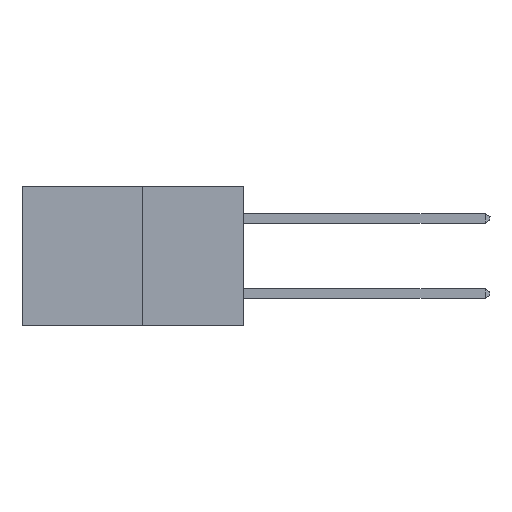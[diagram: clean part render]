
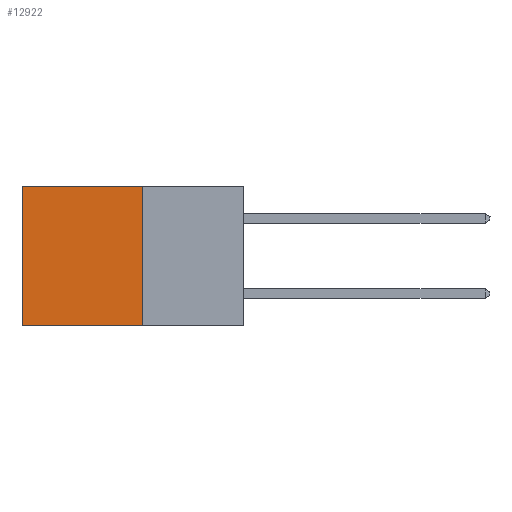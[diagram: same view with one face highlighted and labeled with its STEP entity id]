
A CAD part, left-side view. The second image highlights one B-rep face of the part: STEP entity #12922.
In plain terms, the highlighted planar face has unit normal (-1, 0, 0).
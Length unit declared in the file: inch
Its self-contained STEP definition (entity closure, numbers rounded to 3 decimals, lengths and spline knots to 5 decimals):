
#320 = AXIS2_PLACEMENT_3D ( 'NONE', #5425, #6801, #15968 ) ;
#553 = VERTEX_POINT ( 'NONE', #7725 ) ;
#2190 = CARTESIAN_POINT ( 'NONE',  ( 0.277, 0.27, -0.37 ) ) ;
#2912 = EDGE_CURVE ( 'NONE', #14401, #6390, #11120, .T. ) ;
#3602 = EDGE_CURVE ( 'NONE', #6390, #7229, #11902, .T. ) ;
#4695 = CARTESIAN_POINT ( 'NONE',  ( 0.277, 0.59, -0.37 ) ) ;
#5425 = CARTESIAN_POINT ( 'NONE',  ( 0.277, 0.27, -0.37 ) ) ;
#6149 = CARTESIAN_POINT ( 'NONE',  ( 0.277, 0.59, 0. ) ) ;
#6390 = VERTEX_POINT ( 'NONE', #6149 ) ;
#6801 = DIRECTION ( 'NONE',  ( 1., 0., 0. ) ) ;
#7229 = VERTEX_POINT ( 'NONE', #17225 ) ;
#7598 = VECTOR ( 'NONE', #14761, 39.37008 ) ;
#7725 = CARTESIAN_POINT ( 'NONE',  ( 0.277, 0.27, -0.37 ) ) ;
#7935 = DIRECTION ( 'NONE',  ( 0., 0., -1. ) ) ;
#8779 = VECTOR ( 'NONE', #7935, 39.37008 ) ;
#10907 = LINE ( 'NONE', #2190, #11332 ) ;
#10910 = CARTESIAN_POINT ( 'NONE',  ( 0.277, 0.27, -0.37 ) ) ;
#10996 = EDGE_CURVE ( 'NONE', #553, #7229, #10907, .T. ) ;
#11120 = LINE ( 'NONE', #12433, #7598 ) ;
#11332 = VECTOR ( 'NONE', #11873, 39.37008 ) ;
#11873 = DIRECTION ( 'NONE',  ( 0., 1., 0. ) ) ;
#11902 = LINE ( 'NONE', #4695, #8779 ) ;
#12237 = DIRECTION ( 'NONE',  ( 0., 0., -1. ) ) ;
#12433 = CARTESIAN_POINT ( 'NONE',  ( 0.277, 0.27, 0. ) ) ;
#12922 = ADVANCED_FACE ( 'NONE', ( #17463 ), #13471, .F. ) ;
#13375 = EDGE_LOOP ( 'NONE', ( #14861, #15057, #15729, #15846 ) ) ;
#13471 = PLANE ( 'NONE',  #320 ) ;
#13663 = VECTOR ( 'NONE', #12237, 39.37008 ) ;
#14401 = VERTEX_POINT ( 'NONE', #15503 ) ;
#14481 = LINE ( 'NONE', #10910, #13663 ) ;
#14761 = DIRECTION ( 'NONE',  ( 0., 1., 0. ) ) ;
#14861 = ORIENTED_EDGE ( 'NONE', *, *, #3602, .T. ) ;
#15057 = ORIENTED_EDGE ( 'NONE', *, *, #10996, .F. ) ;
#15503 = CARTESIAN_POINT ( 'NONE',  ( 0.277, 0.27, 0. ) ) ;
#15729 = ORIENTED_EDGE ( 'NONE', *, *, #17577, .F. ) ;
#15846 = ORIENTED_EDGE ( 'NONE', *, *, #2912, .T. ) ;
#15968 = DIRECTION ( 'NONE',  ( 0., 0., -1. ) ) ;
#17225 = CARTESIAN_POINT ( 'NONE',  ( 0.277, 0.59, -0.37 ) ) ;
#17463 = FACE_OUTER_BOUND ( 'NONE', #13375, .T. ) ;
#17577 = EDGE_CURVE ( 'NONE', #14401, #553, #14481, .T. ) ;
